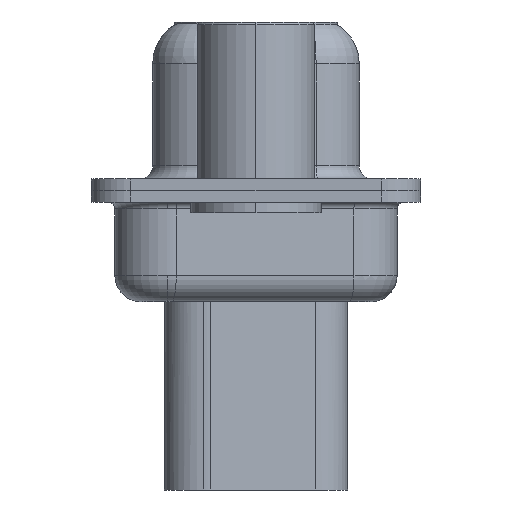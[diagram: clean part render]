
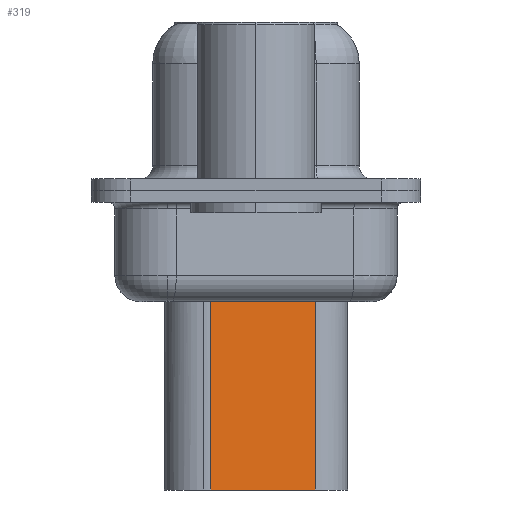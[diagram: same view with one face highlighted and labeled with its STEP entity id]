
A CAD part, left-side view. The second image highlights one B-rep face of the part: STEP entity #319.
In plain terms, the highlighted planar face has unit normal (-0.985, -0.174, 0).
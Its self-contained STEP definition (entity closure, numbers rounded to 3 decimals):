
#319 = ADVANCED_FACE ( 'NONE', ( #7347 ), #16670, .T. ) ;
#754 = VECTOR ( 'NONE', #3491, 1000. ) ;
#1320 = DIRECTION ( 'NONE',  ( -0.174, 0.985, 0. ) ) ;
#1395 = ORIENTED_EDGE ( 'NONE', *, *, #19181, .T. ) ;
#3248 = LINE ( 'NONE', #5530, #11184 ) ;
#3284 = LINE ( 'NONE', #12184, #22064 ) ;
#3491 = DIRECTION ( 'NONE',  ( 0., 0., -1. ) ) ;
#4155 = ORIENTED_EDGE ( 'NONE', *, *, #18161, .T. ) ;
#5530 = CARTESIAN_POINT ( 'NONE',  ( 4.524, 1.74, -11.45 ) ) ;
#5625 = DIRECTION ( 'NONE',  ( -0.985, -0.174, 0. ) ) ;
#5714 = DIRECTION ( 'NONE',  ( 0.174, -0.985, 0. ) ) ;
#7347 = FACE_OUTER_BOUND ( 'NONE', #23603, .T. ) ;
#7372 = DIRECTION ( 'NONE',  ( -0.174, 0.985, 0. ) ) ;
#8789 = VERTEX_POINT ( 'NONE', #19791 ) ;
#8815 = EDGE_CURVE ( 'NONE', #12001, #10509, #20120, .T. ) ;
#9132 = ORIENTED_EDGE ( 'NONE', *, *, #19208, .F. ) ;
#10509 = VERTEX_POINT ( 'NONE', #14351 ) ;
#11184 = VECTOR ( 'NONE', #7372, 1000. ) ;
#12001 = VERTEX_POINT ( 'NONE', #17756 ) ;
#12184 = CARTESIAN_POINT ( 'NONE',  ( 4.353, 2.709, -3.975 ) ) ;
#12304 = LINE ( 'NONE', #20015, #16607 ) ;
#14351 = CARTESIAN_POINT ( 'NONE',  ( 5.229, -2.26, -11.45 ) ) ;
#14498 = DIRECTION ( 'NONE',  ( 0., 0., -1. ) ) ;
#16607 = VECTOR ( 'NONE', #14498, 1000. ) ;
#16670 = PLANE ( 'NONE',  #21311 ) ;
#16746 = CARTESIAN_POINT ( 'NONE',  ( 4.524, 1.74, -3.1 ) ) ;
#17708 = VERTEX_POINT ( 'NONE', #23170 ) ;
#17756 = CARTESIAN_POINT ( 'NONE',  ( 5.229, -2.26, -3.975 ) ) ;
#18161 = EDGE_CURVE ( 'NONE', #12001, #17708, #3284, .T. ) ;
#19181 = EDGE_CURVE ( 'NONE', #17708, #8789, #12304, .T. ) ;
#19208 = EDGE_CURVE ( 'NONE', #10509, #8789, #3248, .T. ) ;
#19791 = CARTESIAN_POINT ( 'NONE',  ( 4.524, 1.74, -11.45 ) ) ;
#19868 = CARTESIAN_POINT ( 'NONE',  ( 5.229, -2.26, -3.1 ) ) ;
#20015 = CARTESIAN_POINT ( 'NONE',  ( 4.524, 1.74, -3.1 ) ) ;
#20120 = LINE ( 'NONE', #19868, #754 ) ;
#21311 = AXIS2_PLACEMENT_3D ( 'NONE', #16746, #5625, #5714 ) ;
#22064 = VECTOR ( 'NONE', #1320, 1000. ) ;
#22307 = ORIENTED_EDGE ( 'NONE', *, *, #8815, .F. ) ;
#23170 = CARTESIAN_POINT ( 'NONE',  ( 4.524, 1.74, -3.975 ) ) ;
#23603 = EDGE_LOOP ( 'NONE', ( #22307, #4155, #1395, #9132 ) ) ;
